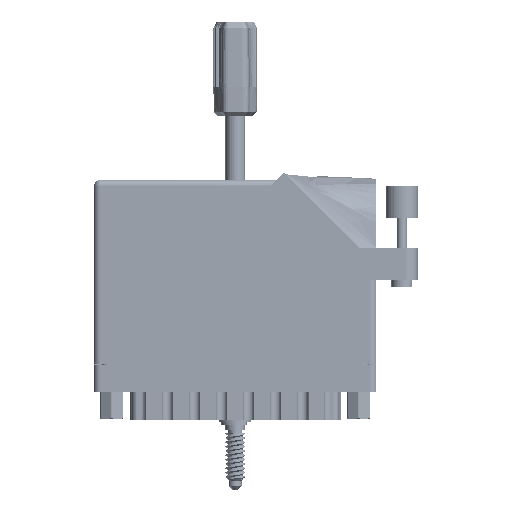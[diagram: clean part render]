
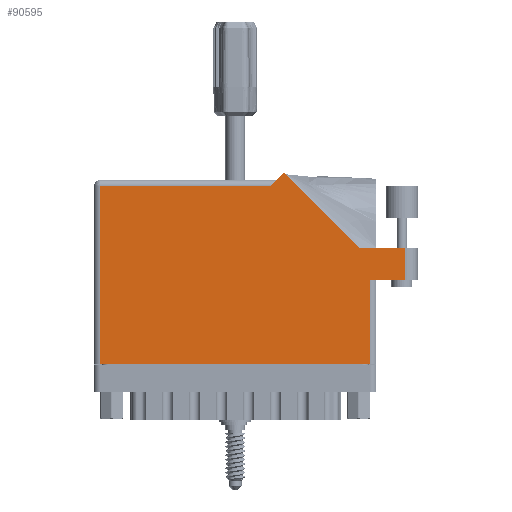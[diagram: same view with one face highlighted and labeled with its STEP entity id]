
A CAD part, front view. The second image highlights one B-rep face of the part: STEP entity #90595.
In plain terms, the highlighted face is planar.
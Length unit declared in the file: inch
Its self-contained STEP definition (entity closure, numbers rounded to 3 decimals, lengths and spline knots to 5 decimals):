
#271 = CARTESIAN_POINT ( 'NONE',  ( 0.062, 0., 0. ) ) ;
#913 = CARTESIAN_POINT ( 'NONE',  ( 0.062, 1.713, 0. ) ) ;
#985 = LINE ( 'NONE', #93305, #17697 ) ;
#1557 = DIRECTION ( 'NONE',  ( 0., 1., 0. ) ) ;
#4557 = CARTESIAN_POINT ( 'NONE',  ( 3.118, 1.122, 0. ) ) ;
#6531 = VECTOR ( 'NONE', #11690, 39.37008 ) ;
#6733 = ORIENTED_EDGE ( 'NONE', *, *, #26179, .T. ) ;
#6924 = ORIENTED_EDGE ( 'NONE', *, *, #91162, .T. ) ;
#11690 = DIRECTION ( 'NONE',  ( 0., 1., 0. ) ) ;
#12005 = CARTESIAN_POINT ( 'NONE',  ( 2.993, 1.122, 0. ) ) ;
#12940 = EDGE_CURVE ( 'NONE', #27787, #94194, #64126, .T. ) ;
#15651 = DIRECTION ( 'NONE',  ( 0., -1., 0. ) ) ;
#15793 = CARTESIAN_POINT ( 'NONE',  ( 0., 0., 0. ) ) ;
#17697 = VECTOR ( 'NONE', #46854, 39.37008 ) ;
#17804 = DIRECTION ( 'NONE',  ( 1., 0., 0. ) ) ;
#20258 = DIRECTION ( 'NONE',  ( -1., 0., 0. ) ) ;
#21588 = EDGE_CURVE ( 'NONE', #42121, #32955, #57135, .T. ) ;
#22551 = DIRECTION ( 'NONE',  ( 0., 0., -1. ) ) ;
#23984 = CARTESIAN_POINT ( 'NONE',  ( 0.062, 0., 0. ) ) ;
#24168 = CARTESIAN_POINT ( 'NONE',  ( 2.656, 0.815, 0. ) ) ;
#24863 = LINE ( 'NONE', #26646, #64239 ) ;
#26115 = CARTESIAN_POINT ( 'NONE',  ( 1.696, 1.713, 0. ) ) ;
#26179 = EDGE_CURVE ( 'NONE', #96586, #27787, #65074, .T. ) ;
#26646 = CARTESIAN_POINT ( 'NONE',  ( 2.55242, 1.122, 0. ) ) ;
#27787 = VERTEX_POINT ( 'NONE', #59966 ) ;
#28493 = FACE_OUTER_BOUND ( 'NONE', #52264, .T. ) ;
#29235 = ORIENTED_EDGE ( 'NONE', *, *, #21588, .T. ) ;
#29533 = VERTEX_POINT ( 'NONE', #26115 ) ;
#30694 = VERTEX_POINT ( 'NONE', #913 ) ;
#31818 = VECTOR ( 'NONE', #20258, 39.37008 ) ;
#32955 = VERTEX_POINT ( 'NONE', #69450 ) ;
#36113 = EDGE_CURVE ( 'NONE', #62701, #96586, #72239, .T. ) ;
#42121 = VERTEX_POINT ( 'NONE', #271 ) ;
#43151 = EDGE_CURVE ( 'NONE', #29533, #30694, #44313, .T. ) ;
#43761 = ORIENTED_EDGE ( 'NONE', *, *, #12940, .T. ) ;
#43985 = ORIENTED_EDGE ( 'NONE', *, *, #43151, .T. ) ;
#44313 = LINE ( 'NONE', #44623, #81383 ) ;
#44623 = CARTESIAN_POINT ( 'NONE',  ( 0., 1.713, 0. ) ) ;
#45529 = DIRECTION ( 'NONE',  ( -1., 0., 0. ) ) ;
#45857 = PLANE ( 'NONE',  #76894 ) ;
#45981 = LINE ( 'NONE', #62635, #69990 ) ;
#46182 = CARTESIAN_POINT ( 'NONE',  ( 0., 1.775, 0. ) ) ;
#46854 = DIRECTION ( 'NONE',  ( -0.707, -0.707, 0. ) ) ;
#52264 = EDGE_LOOP ( 'NONE', ( #79570, #6733, #43761, #6924, #91302, #43985, #66417, #29235, #85534 ) ) ;
#54235 = VECTOR ( 'NONE', #17804, 39.37008 ) ;
#54478 = CARTESIAN_POINT ( 'NONE',  ( 2.718, 0.815, 0. ) ) ;
#57098 = CARTESIAN_POINT ( 'NONE',  ( 2.55242, 1.122, 0. ) ) ;
#57135 = LINE ( 'NONE', #15793, #79927 ) ;
#59966 = CARTESIAN_POINT ( 'NONE',  ( 2.993, 1.122, 0. ) ) ;
#60308 = DIRECTION ( 'NONE',  ( -1., 0., 0. ) ) ;
#62475 = DIRECTION ( 'NONE',  ( 1., 0., 0. ) ) ;
#62635 = CARTESIAN_POINT ( 'NONE',  ( 2.656, 0.815, 0. ) ) ;
#62701 = VERTEX_POINT ( 'NONE', #24168 ) ;
#64126 = LINE ( 'NONE', #4557, #31818 ) ;
#64239 = VECTOR ( 'NONE', #95451, 39.37008 ) ;
#64768 = VECTOR ( 'NONE', #15651, 39.37008 ) ;
#65074 = LINE ( 'NONE', #12005, #6531 ) ;
#66413 = EDGE_CURVE ( 'NONE', #98422, #29533, #985, .T. ) ;
#66417 = ORIENTED_EDGE ( 'NONE', *, *, #77764, .T. ) ;
#68948 = CARTESIAN_POINT ( 'NONE',  ( 1.82871, 1.84571, 0. ) ) ;
#69450 = CARTESIAN_POINT ( 'NONE',  ( 2.656, 0., 0. ) ) ;
#69990 = VECTOR ( 'NONE', #1557, 39.37008 ) ;
#72239 = LINE ( 'NONE', #54478, #54235 ) ;
#74384 = LINE ( 'NONE', #23984, #64768 ) ;
#76894 = AXIS2_PLACEMENT_3D ( 'NONE', #46182, #22551, #45529 ) ;
#77764 = EDGE_CURVE ( 'NONE', #30694, #42121, #74384, .T. ) ;
#79570 = ORIENTED_EDGE ( 'NONE', *, *, #36113, .T. ) ;
#79927 = VECTOR ( 'NONE', #62475, 39.37008 ) ;
#81053 = CARTESIAN_POINT ( 'NONE',  ( 2.993, 0.815, 0. ) ) ;
#81383 = VECTOR ( 'NONE', #60308, 39.37008 ) ;
#83118 = EDGE_CURVE ( 'NONE', #32955, #62701, #45981, .T. ) ;
#85534 = ORIENTED_EDGE ( 'NONE', *, *, #83118, .T. ) ;
#90595 = ADVANCED_FACE ( 'NONE', ( #28493 ), #45857, .F. ) ;
#91162 = EDGE_CURVE ( 'NONE', #94194, #98422, #24863, .T. ) ;
#91302 = ORIENTED_EDGE ( 'NONE', *, *, #66413, .T. ) ;
#93305 = CARTESIAN_POINT ( 'NONE',  ( 1.758, 1.775, 0. ) ) ;
#94194 = VERTEX_POINT ( 'NONE', #57098 ) ;
#95451 = DIRECTION ( 'NONE',  ( -0.707, 0.707, 0. ) ) ;
#96586 = VERTEX_POINT ( 'NONE', #81053 ) ;
#98422 = VERTEX_POINT ( 'NONE', #68948 ) ;
